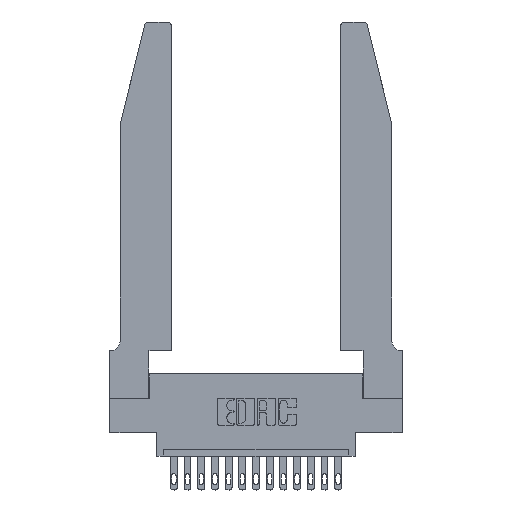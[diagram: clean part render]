
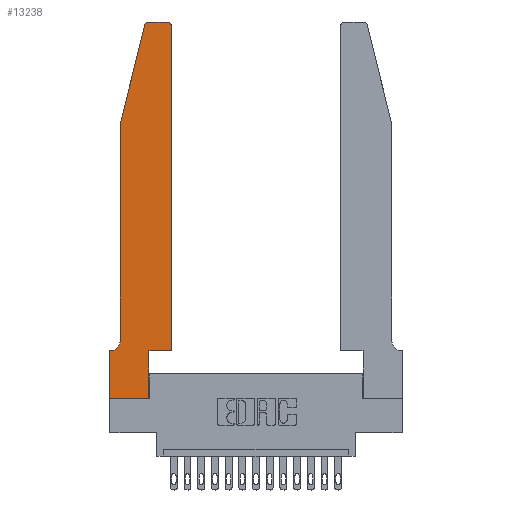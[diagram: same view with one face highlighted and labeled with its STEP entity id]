
A CAD part, top view. The second image highlights one B-rep face of the part: STEP entity #13238.
In plain terms, the highlighted planar face has unit normal (0, 0, 1).
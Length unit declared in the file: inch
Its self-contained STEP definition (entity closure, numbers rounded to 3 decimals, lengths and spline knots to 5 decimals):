
#231 = CIRCLE ( 'NONE', #11430, 0.07 ) ;
#793 = CARTESIAN_POINT ( 'NONE',  ( 0., 0.35, 0.37 ) ) ;
#945 = EDGE_CURVE ( 'NONE', #17613, #15035, #13191, .T. ) ;
#1306 = ORIENTED_EDGE ( 'NONE', *, *, #12257, .T. ) ;
#1370 = LINE ( 'NONE', #16592, #6480 ) ;
#2173 = CARTESIAN_POINT ( 'NONE',  ( 0.0055, 0.35, 0.37 ) ) ;
#2406 = DIRECTION ( 'NONE',  ( 1., 0., 0. ) ) ;
#2411 = EDGE_CURVE ( 'NONE', #4092, #17263, #11551, .T. ) ;
#2546 = DIRECTION ( 'NONE',  ( 1., 0., 0. ) ) ;
#2663 = EDGE_CURVE ( 'NONE', #10890, #17613, #12441, .T. ) ;
#2994 = AXIS2_PLACEMENT_3D ( 'NONE', #3632, #15181, #17741 ) ;
#3054 = ORIENTED_EDGE ( 'NONE', *, *, #945, .T. ) ;
#3073 = VERTEX_POINT ( 'NONE', #9975 ) ;
#3542 = VECTOR ( 'NONE', #17422, 39.37008 ) ;
#3632 = CARTESIAN_POINT ( 'NONE',  ( 0.284, 2.72, 0.37 ) ) ;
#3778 = DIRECTION ( 'NONE',  ( 0., 0., 1. ) ) ;
#4018 = CARTESIAN_POINT ( 'NONE',  ( 0.4505, 0.35, 0.37 ) ) ;
#4092 = VERTEX_POINT ( 'NONE', #5251 ) ;
#4113 = ORIENTED_EDGE ( 'NONE', *, *, #7708, .T. ) ;
#4217 = VERTEX_POINT ( 'NONE', #12621 ) ;
#4373 = DIRECTION ( 'NONE',  ( -0.239, -0.971, 0. ) ) ;
#4498 = CARTESIAN_POINT ( 'NONE',  ( 0.0755, 2., 0.37 ) ) ;
#4719 = FACE_OUTER_BOUND ( 'NONE', #12812, .T. ) ;
#4760 = LINE ( 'NONE', #8040, #16818 ) ;
#4909 = AXIS2_PLACEMENT_3D ( 'NONE', #793, #3778, #18071 ) ;
#5011 = ORIENTED_EDGE ( 'NONE', *, *, #13012, .T. ) ;
#5251 = CARTESIAN_POINT ( 'NONE',  ( 0.284, 2.75, 0.37 ) ) ;
#5310 = VECTOR ( 'NONE', #18311, 39.37008 ) ;
#5451 = CARTESIAN_POINT ( 'NONE',  ( 0.4505, 0.35, 0.37 ) ) ;
#5533 = VECTOR ( 'NONE', #2406, 39.37008 ) ;
#5687 = CARTESIAN_POINT ( 'NONE',  ( 0.2865, 0.35, 0.37 ) ) ;
#5694 = CARTESIAN_POINT ( 'NONE',  ( 0.0755, 2., 0.37 ) ) ;
#5959 = ORIENTED_EDGE ( 'NONE', *, *, #2663, .T. ) ;
#5986 = CARTESIAN_POINT ( 'NONE',  ( 0.25487, 2.72718, 0.37 ) ) ;
#6411 = DIRECTION ( 'NONE',  ( -1., 0., 0. ) ) ;
#6480 = VECTOR ( 'NONE', #13663, 39.37008 ) ;
#7008 = CARTESIAN_POINT ( 'NONE',  ( 0.2605, 2.75, 0.37 ) ) ;
#7128 = VECTOR ( 'NONE', #15330, 39.37008 ) ;
#7269 = EDGE_CURVE ( 'NONE', #3073, #4217, #4760, .T. ) ;
#7472 = EDGE_CURVE ( 'NONE', #15035, #14363, #13232, .T. ) ;
#7708 = EDGE_CURVE ( 'NONE', #10404, #3073, #11429, .T. ) ;
#7821 = VECTOR ( 'NONE', #4373, 39.37008 ) ;
#7884 = CARTESIAN_POINT ( 'NONE',  ( 0.0055, 0.42, 0.37 ) ) ;
#8040 = CARTESIAN_POINT ( 'NONE',  ( 0., 0., 0.37 ) ) ;
#8282 = DIRECTION ( 'NONE',  ( 0., 0., 1. ) ) ;
#8895 = EDGE_CURVE ( 'NONE', #10292, #10404, #231, .T. ) ;
#9001 = DIRECTION ( 'NONE',  ( 0., 1., 0. ) ) ;
#9676 = CARTESIAN_POINT ( 'NONE',  ( 0.2865, 0.35, 0.37 ) ) ;
#9914 = EDGE_CURVE ( 'NONE', #14363, #4092, #11336, .T. ) ;
#9975 = CARTESIAN_POINT ( 'NONE',  ( 0., 0.35, 0.37 ) ) ;
#10292 = VERTEX_POINT ( 'NONE', #10669 ) ;
#10343 = ORIENTED_EDGE ( 'NONE', *, *, #8895, .T. ) ;
#10404 = VERTEX_POINT ( 'NONE', #2173 ) ;
#10408 = PLANE ( 'NONE',  #4909 ) ;
#10464 = ORIENTED_EDGE ( 'NONE', *, *, #7269, .T. ) ;
#10634 = DIRECTION ( 'NONE',  ( 0., 0., -1. ) ) ;
#10669 = CARTESIAN_POINT ( 'NONE',  ( 0.0755, 0.42, 0.37 ) ) ;
#10793 = CARTESIAN_POINT ( 'NONE',  ( 0.4205, 2.75, 0.37 ) ) ;
#10890 = VERTEX_POINT ( 'NONE', #9676 ) ;
#10896 = ORIENTED_EDGE ( 'NONE', *, *, #9914, .T. ) ;
#11113 = CARTESIAN_POINT ( 'NONE',  ( 0.2865, 0., 0.37 ) ) ;
#11336 = LINE ( 'NONE', #7008, #5310 ) ;
#11429 = LINE ( 'NONE', #14248, #15696 ) ;
#11430 = AXIS2_PLACEMENT_3D ( 'NONE', #7884, #10634, #14836 ) ;
#11551 = CIRCLE ( 'NONE', #2994, 0.03 ) ;
#12257 = EDGE_CURVE ( 'NONE', #17263, #14903, #13449, .T. ) ;
#12441 = LINE ( 'NONE', #14851, #5533 ) ;
#12621 = CARTESIAN_POINT ( 'NONE',  ( 0., 0., 0.37 ) ) ;
#12812 = EDGE_LOOP ( 'NONE', ( #10896, #14090, #1306, #13258, #10343, #4113, #10464, #13928, #5011, #5959, #3054, #15882 ) ) ;
#13012 = EDGE_CURVE ( 'NONE', #14541, #10890, #13215, .T. ) ;
#13191 = LINE ( 'NONE', #5451, #7128 ) ;
#13215 = LINE ( 'NONE', #5687, #13666 ) ;
#13232 = CIRCLE ( 'NONE', #17647, 0.03 ) ;
#13238 = ADVANCED_FACE ( 'NONE', ( #4719 ), #10408, .T. ) ;
#13258 = ORIENTED_EDGE ( 'NONE', *, *, #14798, .T. ) ;
#13449 = LINE ( 'NONE', #5694, #7821 ) ;
#13453 = EDGE_CURVE ( 'NONE', #4217, #14541, #1370, .T. ) ;
#13663 = DIRECTION ( 'NONE',  ( 1., 0., 0. ) ) ;
#13666 = VECTOR ( 'NONE', #9001, 39.37008 ) ;
#13928 = ORIENTED_EDGE ( 'NONE', *, *, #13453, .T. ) ;
#14090 = ORIENTED_EDGE ( 'NONE', *, *, #2411, .T. ) ;
#14248 = CARTESIAN_POINT ( 'NONE',  ( 0.0755, 0.35, 0.37 ) ) ;
#14363 = VERTEX_POINT ( 'NONE', #10793 ) ;
#14541 = VERTEX_POINT ( 'NONE', #11113 ) ;
#14668 = CARTESIAN_POINT ( 'NONE',  ( 0.0755, 2., 0.37 ) ) ;
#14732 = CARTESIAN_POINT ( 'NONE',  ( 0.4505, 2.72, 0.37 ) ) ;
#14798 = EDGE_CURVE ( 'NONE', #14903, #10292, #17823, .T. ) ;
#14836 = DIRECTION ( 'NONE',  ( -1., 0., 0. ) ) ;
#14851 = CARTESIAN_POINT ( 'NONE',  ( 0.4505, 0.35, 0.37 ) ) ;
#14903 = VERTEX_POINT ( 'NONE', #14668 ) ;
#15035 = VERTEX_POINT ( 'NONE', #14732 ) ;
#15181 = DIRECTION ( 'NONE',  ( 0., 0., 1. ) ) ;
#15330 = DIRECTION ( 'NONE',  ( 0., 1., 0. ) ) ;
#15696 = VECTOR ( 'NONE', #6411, 39.37008 ) ;
#15882 = ORIENTED_EDGE ( 'NONE', *, *, #7472, .T. ) ;
#16592 = CARTESIAN_POINT ( 'NONE',  ( 0., 0., 0.37 ) ) ;
#16818 = VECTOR ( 'NONE', #18040, 39.37008 ) ;
#17042 = CARTESIAN_POINT ( 'NONE',  ( 0.4205, 2.72, 0.37 ) ) ;
#17263 = VERTEX_POINT ( 'NONE', #5986 ) ;
#17422 = DIRECTION ( 'NONE',  ( 0., -1., 0. ) ) ;
#17613 = VERTEX_POINT ( 'NONE', #4018 ) ;
#17647 = AXIS2_PLACEMENT_3D ( 'NONE', #17042, #8282, #2546 ) ;
#17741 = DIRECTION ( 'NONE',  ( 1., 0., 0. ) ) ;
#17823 = LINE ( 'NONE', #4498, #3542 ) ;
#18040 = DIRECTION ( 'NONE',  ( 0., -1., 0. ) ) ;
#18071 = DIRECTION ( 'NONE',  ( 1., 0., 0. ) ) ;
#18311 = DIRECTION ( 'NONE',  ( -1., 0., 0. ) ) ;
